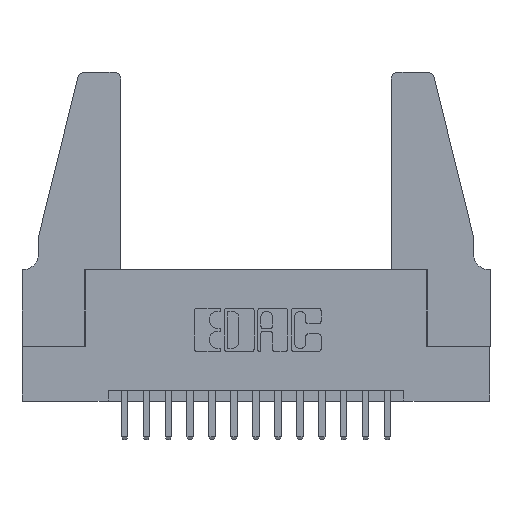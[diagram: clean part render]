
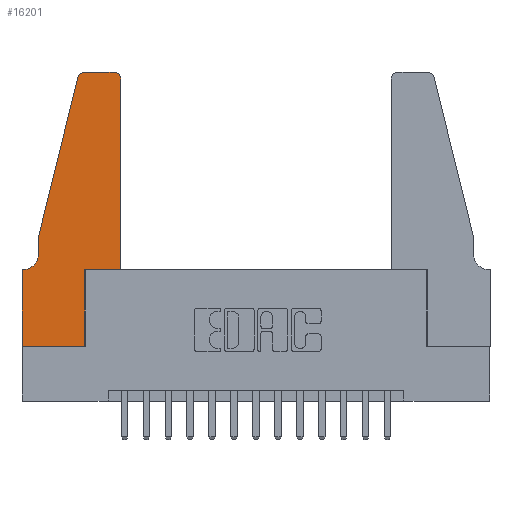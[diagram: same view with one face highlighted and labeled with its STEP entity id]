
A CAD part, top view. The second image highlights one B-rep face of the part: STEP entity #16201.
In plain terms, the highlighted planar face has unit normal (0, 0, 1).
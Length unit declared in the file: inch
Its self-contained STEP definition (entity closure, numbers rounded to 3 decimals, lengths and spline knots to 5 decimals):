
#215 = CARTESIAN_POINT ( 'NONE',  ( 0.0755, 0.5, 0.37 ) ) ;
#260 = DIRECTION ( 'NONE',  ( -1., 0., 0. ) ) ;
#521 = CARTESIAN_POINT ( 'NONE',  ( 0.4205, 1.22, 0.37 ) ) ;
#527 = CARTESIAN_POINT ( 'NONE',  ( 0.284, 1.25, 0.37 ) ) ;
#558 = CARTESIAN_POINT ( 'NONE',  ( 0.2865, 0., 0.37 ) ) ;
#880 = EDGE_CURVE ( 'NONE', #4101, #11141, #3600, .T. ) ;
#901 = CARTESIAN_POINT ( 'NONE',  ( 0.0755, 0.42, 0.37 ) ) ;
#1066 = ORIENTED_EDGE ( 'NONE', *, *, #16140, .T. ) ;
#1139 = CARTESIAN_POINT ( 'NONE',  ( 0.0755, 0.35, 0.37 ) ) ;
#1153 = ORIENTED_EDGE ( 'NONE', *, *, #13919, .T. ) ;
#1166 = AXIS2_PLACEMENT_3D ( 'NONE', #15347, #2840, #12939 ) ;
#1301 = CARTESIAN_POINT ( 'NONE',  ( 0., 0., 0.37 ) ) ;
#1314 = EDGE_CURVE ( 'NONE', #5835, #5366, #9303, .T. ) ;
#1630 = CARTESIAN_POINT ( 'NONE',  ( 0.0755, 0.5, 0.37 ) ) ;
#1720 = DIRECTION ( 'NONE',  ( 1., 0., 0. ) ) ;
#1883 = DIRECTION ( 'NONE',  ( 1., 0., 0. ) ) ;
#1896 = VECTOR ( 'NONE', #5955, 39.37008 ) ;
#1921 = VERTEX_POINT ( 'NONE', #901 ) ;
#1936 = CARTESIAN_POINT ( 'NONE',  ( 0.4505, 1.22, 0.37 ) ) ;
#2176 = VECTOR ( 'NONE', #4449, 39.37008 ) ;
#2334 = LINE ( 'NONE', #215, #5875 ) ;
#2396 = ORIENTED_EDGE ( 'NONE', *, *, #9778, .T. ) ;
#2446 = VERTEX_POINT ( 'NONE', #558 ) ;
#2738 = LINE ( 'NONE', #3859, #8461 ) ;
#2840 = DIRECTION ( 'NONE',  ( 0., 0., 1. ) ) ;
#2881 = ORIENTED_EDGE ( 'NONE', *, *, #9710, .T. ) ;
#3088 = CARTESIAN_POINT ( 'NONE',  ( 0.4505, 0.35, 0.37 ) ) ;
#3145 = CARTESIAN_POINT ( 'NONE',  ( 0., 0.35, 0.37 ) ) ;
#3178 = ORIENTED_EDGE ( 'NONE', *, *, #11747, .T. ) ;
#3600 = LINE ( 'NONE', #1139, #9532 ) ;
#3765 = CARTESIAN_POINT ( 'NONE',  ( 0.2865, 0.35, 0.37 ) ) ;
#3857 = LINE ( 'NONE', #9721, #1896 ) ;
#3859 = CARTESIAN_POINT ( 'NONE',  ( 0.4505, 0.35, 0.37 ) ) ;
#3887 = CARTESIAN_POINT ( 'NONE',  ( 0.0055, 0.35, 0.37 ) ) ;
#4007 = VECTOR ( 'NONE', #12975, 39.37008 ) ;
#4053 = PLANE ( 'NONE',  #1166 ) ;
#4091 = DIRECTION ( 'NONE',  ( 0., -1., 0. ) ) ;
#4101 = VERTEX_POINT ( 'NONE', #3887 ) ;
#4449 = DIRECTION ( 'NONE',  ( 0., 1., 0. ) ) ;
#5148 = CARTESIAN_POINT ( 'NONE',  ( 0.4205, 1.25, 0.37 ) ) ;
#5193 = LINE ( 'NONE', #14226, #4007 ) ;
#5207 = CARTESIAN_POINT ( 'NONE',  ( 0.4505, 0.35, 0.37 ) ) ;
#5299 = ORIENTED_EDGE ( 'NONE', *, *, #1314, .T. ) ;
#5366 = VERTEX_POINT ( 'NONE', #527 ) ;
#5657 = LINE ( 'NONE', #1630, #7037 ) ;
#5746 = VERTEX_POINT ( 'NONE', #11724 ) ;
#5776 = CARTESIAN_POINT ( 'NONE',  ( 0.25487, 1.22718, 0.37 ) ) ;
#5835 = VERTEX_POINT ( 'NONE', #5148 ) ;
#5875 = VECTOR ( 'NONE', #4091, 39.37008 ) ;
#5936 = VECTOR ( 'NONE', #260, 39.37008 ) ;
#5955 = DIRECTION ( 'NONE',  ( 0., 1., 0. ) ) ;
#6146 = VERTEX_POINT ( 'NONE', #5776 ) ;
#6687 = DIRECTION ( 'NONE',  ( -0.239, -0.971, 0. ) ) ;
#6844 = EDGE_LOOP ( 'NONE', ( #5299, #1153, #10958, #14945, #2881, #11080, #10806, #1066, #15455, #3178, #8011, #2396 ) ) ;
#7037 = VECTOR ( 'NONE', #6687, 39.37008 ) ;
#7483 = LINE ( 'NONE', #3088, #2176 ) ;
#7791 = CIRCLE ( 'NONE', #8294, 0.03 ) ;
#8011 = ORIENTED_EDGE ( 'NONE', *, *, #11149, .T. ) ;
#8201 = DIRECTION ( 'NONE',  ( -1., 0., 0. ) ) ;
#8233 = EDGE_CURVE ( 'NONE', #11141, #12133, #5193, .T. ) ;
#8294 = AXIS2_PLACEMENT_3D ( 'NONE', #9875, #14980, #8651 ) ;
#8308 = VERTEX_POINT ( 'NONE', #1936 ) ;
#8461 = VECTOR ( 'NONE', #1720, 39.37008 ) ;
#8651 = DIRECTION ( 'NONE',  ( 1., 0., 0. ) ) ;
#8674 = DIRECTION ( 'NONE',  ( -1., 0., 0. ) ) ;
#8731 = LINE ( 'NONE', #1301, #9519 ) ;
#9303 = LINE ( 'NONE', #10504, #5936 ) ;
#9317 = DIRECTION ( 'NONE',  ( 0., 0., -1. ) ) ;
#9432 = DIRECTION ( 'NONE',  ( 0., 0., 1. ) ) ;
#9519 = VECTOR ( 'NONE', #15060, 39.37008 ) ;
#9532 = VECTOR ( 'NONE', #8674, 39.37008 ) ;
#9710 = EDGE_CURVE ( 'NONE', #1921, #4101, #10668, .T. ) ;
#9721 = CARTESIAN_POINT ( 'NONE',  ( 0.2865, 0.35, 0.37 ) ) ;
#9778 = EDGE_CURVE ( 'NONE', #8308, #5835, #11643, .T. ) ;
#9875 = CARTESIAN_POINT ( 'NONE',  ( 0.284, 1.22, 0.37 ) ) ;
#10504 = CARTESIAN_POINT ( 'NONE',  ( 0.2605, 1.25, 0.37 ) ) ;
#10668 = CIRCLE ( 'NONE', #15843, 0.07 ) ;
#10806 = ORIENTED_EDGE ( 'NONE', *, *, #8233, .T. ) ;
#10958 = ORIENTED_EDGE ( 'NONE', *, *, #13113, .T. ) ;
#11080 = ORIENTED_EDGE ( 'NONE', *, *, #880, .T. ) ;
#11141 = VERTEX_POINT ( 'NONE', #3145 ) ;
#11149 = EDGE_CURVE ( 'NONE', #12349, #8308, #7483, .T. ) ;
#11279 = FACE_OUTER_BOUND ( 'NONE', #6844, .T. ) ;
#11643 = CIRCLE ( 'NONE', #13378, 0.03 ) ;
#11724 = CARTESIAN_POINT ( 'NONE',  ( 0.0755, 0.5, 0.37 ) ) ;
#11747 = EDGE_CURVE ( 'NONE', #14839, #12349, #2738, .T. ) ;
#12133 = VERTEX_POINT ( 'NONE', #15474 ) ;
#12172 = EDGE_CURVE ( 'NONE', #5746, #1921, #2334, .T. ) ;
#12349 = VERTEX_POINT ( 'NONE', #5207 ) ;
#12939 = DIRECTION ( 'NONE',  ( 1., 0., 0. ) ) ;
#12975 = DIRECTION ( 'NONE',  ( 0., -1., 0. ) ) ;
#13113 = EDGE_CURVE ( 'NONE', #6146, #5746, #5657, .T. ) ;
#13207 = CARTESIAN_POINT ( 'NONE',  ( 0.0055, 0.42, 0.37 ) ) ;
#13378 = AXIS2_PLACEMENT_3D ( 'NONE', #521, #9432, #1883 ) ;
#13407 = EDGE_CURVE ( 'NONE', #2446, #14839, #3857, .T. ) ;
#13919 = EDGE_CURVE ( 'NONE', #5366, #6146, #7791, .T. ) ;
#14226 = CARTESIAN_POINT ( 'NONE',  ( 0., 0., 0.37 ) ) ;
#14839 = VERTEX_POINT ( 'NONE', #3765 ) ;
#14945 = ORIENTED_EDGE ( 'NONE', *, *, #12172, .T. ) ;
#14980 = DIRECTION ( 'NONE',  ( 0., 0., 1. ) ) ;
#15060 = DIRECTION ( 'NONE',  ( 1., 0., 0. ) ) ;
#15347 = CARTESIAN_POINT ( 'NONE',  ( 0., 0.35, 0.37 ) ) ;
#15455 = ORIENTED_EDGE ( 'NONE', *, *, #13407, .T. ) ;
#15474 = CARTESIAN_POINT ( 'NONE',  ( 0., 0., 0.37 ) ) ;
#15843 = AXIS2_PLACEMENT_3D ( 'NONE', #13207, #9317, #8201 ) ;
#16140 = EDGE_CURVE ( 'NONE', #12133, #2446, #8731, .T. ) ;
#16201 = ADVANCED_FACE ( 'NONE', ( #11279 ), #4053, .T. ) ;
